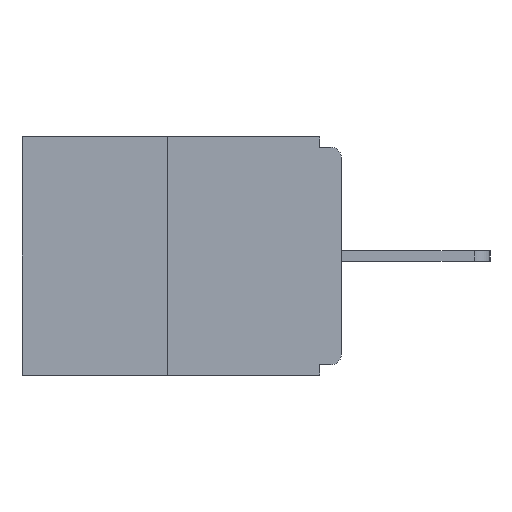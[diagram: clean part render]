
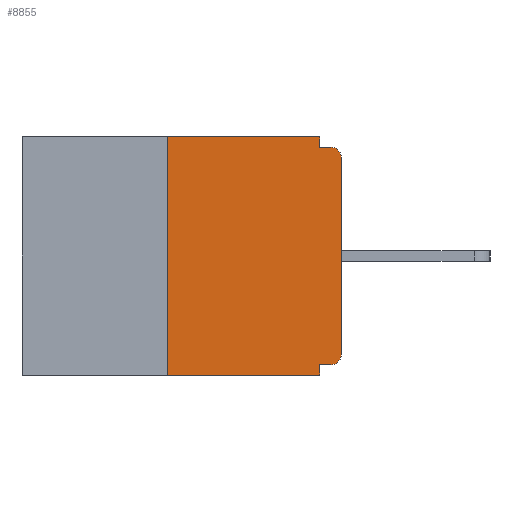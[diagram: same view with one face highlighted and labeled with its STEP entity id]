
A CAD part, left-side view. The second image highlights one B-rep face of the part: STEP entity #8855.
In plain terms, the highlighted planar face has unit normal (-1, 0, 0).
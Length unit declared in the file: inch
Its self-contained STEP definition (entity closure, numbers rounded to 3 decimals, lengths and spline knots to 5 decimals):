
#43 = CARTESIAN_POINT ( 'NONE',  ( 0., 0.015, -0.015 ) ) ;
#124 = CIRCLE ( 'NONE', #8288, 0.015 ) ;
#205 = VERTEX_POINT ( 'NONE', #9066 ) ;
#453 = LINE ( 'NONE', #14277, #1727 ) ;
#706 = DIRECTION ( 'NONE',  ( -1., 0., 0. ) ) ;
#778 = ORIENTED_EDGE ( 'NONE', *, *, #14543, .T. ) ;
#810 = VERTEX_POINT ( 'NONE', #15110 ) ;
#1305 = EDGE_CURVE ( 'NONE', #4252, #205, #9401, .T. ) ;
#1424 = LINE ( 'NONE', #15085, #7311 ) ;
#1727 = VECTOR ( 'NONE', #8944, 39.37008 ) ;
#1867 = DIRECTION ( 'NONE',  ( 0., 1., 0. ) ) ;
#2046 = VECTOR ( 'NONE', #11101, 39.37008 ) ;
#2228 = EDGE_LOOP ( 'NONE', ( #7388, #8872, #6915, #10613, #11253, #7361, #778, #11788, #2497, #4742 ) ) ;
#2377 = VERTEX_POINT ( 'NONE', #4266 ) ;
#2497 = ORIENTED_EDGE ( 'NONE', *, *, #6674, .F. ) ;
#2991 = DIRECTION ( 'NONE',  ( 0., -1., 0. ) ) ;
#3168 = CARTESIAN_POINT ( 'NONE',  ( 0., 0.015, -0.313 ) ) ;
#3525 = EDGE_CURVE ( 'NONE', #810, #6126, #124, .T. ) ;
#3579 = CARTESIAN_POINT ( 'NONE',  ( 0., 0.25, 0. ) ) ;
#3631 = LINE ( 'NONE', #16192, #2046 ) ;
#4147 = VERTEX_POINT ( 'NONE', #12528 ) ;
#4252 = VERTEX_POINT ( 'NONE', #3579 ) ;
#4266 = CARTESIAN_POINT ( 'NONE',  ( 0., 0., -0.313 ) ) ;
#4465 = VECTOR ( 'NONE', #5886, 39.37008 ) ;
#4580 = CARTESIAN_POINT ( 'NONE',  ( 0., 0.015, -0.03 ) ) ;
#4615 = VECTOR ( 'NONE', #10796, 39.37008 ) ;
#4742 = ORIENTED_EDGE ( 'NONE', *, *, #12812, .F. ) ;
#5457 = VECTOR ( 'NONE', #1867, 39.37008 ) ;
#5564 = LINE ( 'NONE', #9248, #6275 ) ;
#5622 = LINE ( 'NONE', #14322, #6544 ) ;
#5654 = CARTESIAN_POINT ( 'NONE',  ( 0., 0.46, 0. ) ) ;
#5745 = CARTESIAN_POINT ( 'NONE',  ( 0., 0., -0.328 ) ) ;
#5813 = LINE ( 'NONE', #14587, #4465 ) ;
#5886 = DIRECTION ( 'NONE',  ( 0., -1., 0. ) ) ;
#5910 = EDGE_CURVE ( 'NONE', #14178, #10710, #13050, .T. ) ;
#6019 = CIRCLE ( 'NONE', #7329, 0.015 ) ;
#6126 = VERTEX_POINT ( 'NONE', #43 ) ;
#6223 = EDGE_CURVE ( 'NONE', #9415, #4252, #1424, .T. ) ;
#6275 = VECTOR ( 'NONE', #14431, 39.37008 ) ;
#6361 = EDGE_CURVE ( 'NONE', #10710, #4147, #5564, .T. ) ;
#6544 = VECTOR ( 'NONE', #2991, 39.37008 ) ;
#6674 = EDGE_CURVE ( 'NONE', #13123, #6126, #5622, .T. ) ;
#6887 = PLANE ( 'NONE',  #7867 ) ;
#6915 = ORIENTED_EDGE ( 'NONE', *, *, #7680, .T. ) ;
#7311 = VECTOR ( 'NONE', #11479, 39.37008 ) ;
#7329 = AXIS2_PLACEMENT_3D ( 'NONE', #3168, #10550, #8191 ) ;
#7361 = ORIENTED_EDGE ( 'NONE', *, *, #15158, .T. ) ;
#7388 = ORIENTED_EDGE ( 'NONE', *, *, #1305, .F. ) ;
#7680 = EDGE_CURVE ( 'NONE', #9415, #4147, #5813, .T. ) ;
#7867 = AXIS2_PLACEMENT_3D ( 'NONE', #5654, #10653, #15676 ) ;
#8191 = DIRECTION ( 'NONE',  ( 0., 0., -1. ) ) ;
#8288 = AXIS2_PLACEMENT_3D ( 'NONE', #4580, #706, #14526 ) ;
#8561 = CARTESIAN_POINT ( 'NONE',  ( 0., 0.25, -0.343 ) ) ;
#8855 = ADVANCED_FACE ( 'NONE', ( #13130 ), #6887, .F. ) ;
#8872 = ORIENTED_EDGE ( 'NONE', *, *, #6223, .F. ) ;
#8944 = DIRECTION ( 'NONE',  ( 0., 0., -1. ) ) ;
#9066 = CARTESIAN_POINT ( 'NONE',  ( 0., 0.031, 0. ) ) ;
#9248 = CARTESIAN_POINT ( 'NONE',  ( 0., 0.031, -0.343 ) ) ;
#9401 = LINE ( 'NONE', #9651, #4615 ) ;
#9415 = VERTEX_POINT ( 'NONE', #8561 ) ;
#9651 = CARTESIAN_POINT ( 'NONE',  ( 0., 0.46, 0. ) ) ;
#10444 = CARTESIAN_POINT ( 'NONE',  ( 0., 0.015, -0.328 ) ) ;
#10550 = DIRECTION ( 'NONE',  ( -1., 0., 0. ) ) ;
#10613 = ORIENTED_EDGE ( 'NONE', *, *, #6361, .F. ) ;
#10653 = DIRECTION ( 'NONE',  ( 1., 0., 0. ) ) ;
#10710 = VERTEX_POINT ( 'NONE', #12515 ) ;
#10796 = DIRECTION ( 'NONE',  ( 0., -1., 0. ) ) ;
#11101 = DIRECTION ( 'NONE',  ( 0., 0., 1. ) ) ;
#11253 = ORIENTED_EDGE ( 'NONE', *, *, #5910, .F. ) ;
#11479 = DIRECTION ( 'NONE',  ( 0., 0., 1. ) ) ;
#11788 = ORIENTED_EDGE ( 'NONE', *, *, #3525, .T. ) ;
#12515 = CARTESIAN_POINT ( 'NONE',  ( 0., 0.031, -0.328 ) ) ;
#12528 = CARTESIAN_POINT ( 'NONE',  ( 0., 0.031, -0.343 ) ) ;
#12812 = EDGE_CURVE ( 'NONE', #205, #13123, #453, .T. ) ;
#13050 = LINE ( 'NONE', #5745, #5457 ) ;
#13123 = VERTEX_POINT ( 'NONE', #15928 ) ;
#13130 = FACE_OUTER_BOUND ( 'NONE', #2228, .T. ) ;
#14178 = VERTEX_POINT ( 'NONE', #10444 ) ;
#14277 = CARTESIAN_POINT ( 'NONE',  ( 0., 0.031, 0. ) ) ;
#14322 = CARTESIAN_POINT ( 'NONE',  ( 0., 0., -0.015 ) ) ;
#14431 = DIRECTION ( 'NONE',  ( 0., 0., -1. ) ) ;
#14526 = DIRECTION ( 'NONE',  ( 0., 0., -1. ) ) ;
#14543 = EDGE_CURVE ( 'NONE', #2377, #810, #3631, .T. ) ;
#14587 = CARTESIAN_POINT ( 'NONE',  ( 0., 0.46, -0.343 ) ) ;
#15085 = CARTESIAN_POINT ( 'NONE',  ( 0., 0.25, 0. ) ) ;
#15110 = CARTESIAN_POINT ( 'NONE',  ( 0., 0., -0.03 ) ) ;
#15158 = EDGE_CURVE ( 'NONE', #14178, #2377, #6019, .T. ) ;
#15676 = DIRECTION ( 'NONE',  ( 0., 0., -1. ) ) ;
#15928 = CARTESIAN_POINT ( 'NONE',  ( 0., 0.031, -0.015 ) ) ;
#16192 = CARTESIAN_POINT ( 'NONE',  ( 0., 0., 0. ) ) ;
